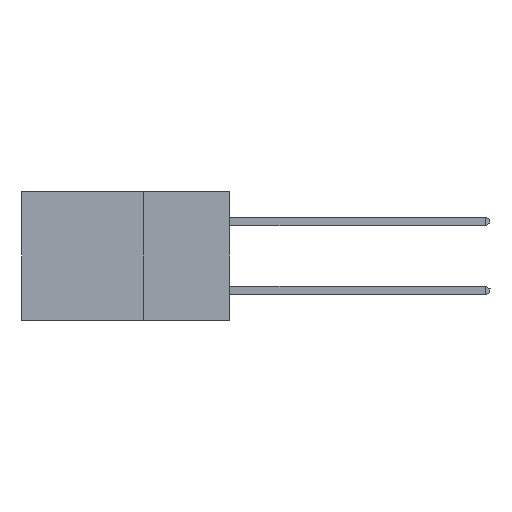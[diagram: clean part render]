
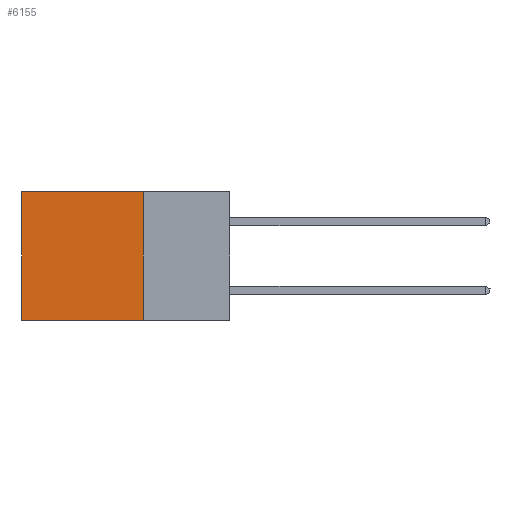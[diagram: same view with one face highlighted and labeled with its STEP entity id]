
A CAD part, left-side view. The second image highlights one B-rep face of the part: STEP entity #6155.
In plain terms, the highlighted planar face has unit normal (-1, 0, 0).
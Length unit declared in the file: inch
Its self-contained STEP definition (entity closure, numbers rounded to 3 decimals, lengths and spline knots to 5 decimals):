
#606 = VECTOR ( 'NONE', #7060, 39.37008 ) ;
#710 = EDGE_CURVE ( 'NONE', #5761, #21459, #10693, .T. ) ;
#1493 = DIRECTION ( 'NONE',  ( 0., 0., -1. ) ) ;
#2001 = EDGE_LOOP ( 'NONE', ( #18776, #15361, #21573, #20611 ) ) ;
#3332 = VECTOR ( 'NONE', #15231, 39.37008 ) ;
#3419 = LINE ( 'NONE', #12644, #606 ) ;
#5761 = VERTEX_POINT ( 'NONE', #14722 ) ;
#5796 = VERTEX_POINT ( 'NONE', #10339 ) ;
#6155 = ADVANCED_FACE ( 'NONE', ( #27642 ), #12646, .F. ) ;
#6456 = CARTESIAN_POINT ( 'NONE',  ( 0.298, 0.25, -0.37 ) ) ;
#7060 = DIRECTION ( 'NONE',  ( 0., 0., -1. ) ) ;
#9979 = LINE ( 'NONE', #10289, #12396 ) ;
#10114 = CARTESIAN_POINT ( 'NONE',  ( 0.298, 0.25, 0. ) ) ;
#10289 = CARTESIAN_POINT ( 'NONE',  ( 0.298, 0.6, 0. ) ) ;
#10339 = CARTESIAN_POINT ( 'NONE',  ( 0.298, 0.6, 0. ) ) ;
#10343 = AXIS2_PLACEMENT_3D ( 'NONE', #28387, #14890, #1493 ) ;
#10693 = LINE ( 'NONE', #6456, #3332 ) ;
#10902 = DIRECTION ( 'NONE',  ( 0., 1., 0. ) ) ;
#11481 = EDGE_CURVE ( 'NONE', #19556, #5796, #14541, .T. ) ;
#12396 = VECTOR ( 'NONE', #17017, 39.37008 ) ;
#12644 = CARTESIAN_POINT ( 'NONE',  ( 0.298, 0.25, 0. ) ) ;
#12646 = PLANE ( 'NONE',  #10343 ) ;
#12916 = CARTESIAN_POINT ( 'NONE',  ( 0.298, 0.25, 0. ) ) ;
#13251 = CARTESIAN_POINT ( 'NONE',  ( 0.298, 0.6, -0.37 ) ) ;
#13593 = EDGE_CURVE ( 'NONE', #19556, #5761, #3419, .T. ) ;
#14541 = LINE ( 'NONE', #12916, #19793 ) ;
#14722 = CARTESIAN_POINT ( 'NONE',  ( 0.298, 0.25, -0.37 ) ) ;
#14890 = DIRECTION ( 'NONE',  ( 1., 0., 0. ) ) ;
#15231 = DIRECTION ( 'NONE',  ( 0., 1., 0. ) ) ;
#15361 = ORIENTED_EDGE ( 'NONE', *, *, #710, .F. ) ;
#17017 = DIRECTION ( 'NONE',  ( 0., 0., -1. ) ) ;
#18776 = ORIENTED_EDGE ( 'NONE', *, *, #22975, .T. ) ;
#19556 = VERTEX_POINT ( 'NONE', #10114 ) ;
#19793 = VECTOR ( 'NONE', #10902, 39.37008 ) ;
#20611 = ORIENTED_EDGE ( 'NONE', *, *, #11481, .T. ) ;
#21459 = VERTEX_POINT ( 'NONE', #13251 ) ;
#21573 = ORIENTED_EDGE ( 'NONE', *, *, #13593, .F. ) ;
#22975 = EDGE_CURVE ( 'NONE', #5796, #21459, #9979, .T. ) ;
#27642 = FACE_OUTER_BOUND ( 'NONE', #2001, .T. ) ;
#28387 = CARTESIAN_POINT ( 'NONE',  ( 0.298, 0.25, 0. ) ) ;
